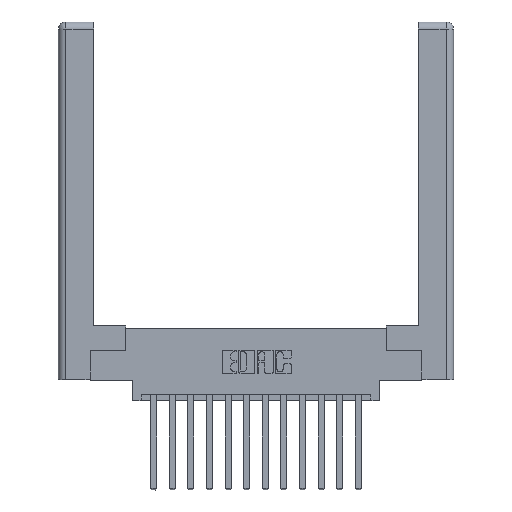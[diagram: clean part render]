
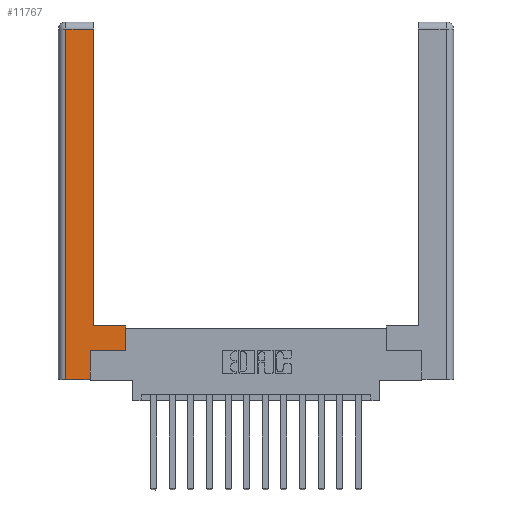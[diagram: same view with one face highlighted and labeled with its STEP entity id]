
A CAD part, top view. The second image highlights one B-rep face of the part: STEP entity #11767.
In plain terms, the highlighted planar face has unit normal (0, 0, 1).
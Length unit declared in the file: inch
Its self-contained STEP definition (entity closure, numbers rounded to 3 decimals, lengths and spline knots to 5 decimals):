
#79 = CARTESIAN_POINT ( 'NONE',  ( 0.265, 0.245, 0. ) ) ;
#194 = CARTESIAN_POINT ( 'NONE',  ( 0.295, 0.45, 0. ) ) ;
#247 = LINE ( 'NONE', #12439, #4839 ) ;
#283 = DIRECTION ( 'NONE',  ( -1., 0., 0. ) ) ;
#370 = LINE ( 'NONE', #435, #12954 ) ;
#431 = ORIENTED_EDGE ( 'NONE', *, *, #11980, .T. ) ;
#435 = CARTESIAN_POINT ( 'NONE',  ( 0.295, 3., 0. ) ) ;
#1293 = CARTESIAN_POINT ( 'NONE',  ( 0.565, 0.45, 0. ) ) ;
#1316 = CARTESIAN_POINT ( 'NONE',  ( 0.565, 0.245, 0. ) ) ;
#1406 = PLANE ( 'NONE',  #14299 ) ;
#1711 = VERTEX_POINT ( 'NONE', #15474 ) ;
#1734 = VERTEX_POINT ( 'NONE', #9394 ) ;
#1900 = CARTESIAN_POINT ( 'NONE',  ( 0.0615, 0., 0. ) ) ;
#2118 = CARTESIAN_POINT ( 'NONE',  ( 0.0615, 2.94, 0. ) ) ;
#2550 = DIRECTION ( 'NONE',  ( 1., 0., 0. ) ) ;
#3252 = CARTESIAN_POINT ( 'NONE',  ( 0.295, 2.94, 0. ) ) ;
#3367 = EDGE_CURVE ( 'NONE', #1734, #9697, #247, .T. ) ;
#4539 = VECTOR ( 'NONE', #8181, 39.37008 ) ;
#4839 = VECTOR ( 'NONE', #6400, 39.37008 ) ;
#5872 = VERTEX_POINT ( 'NONE', #3252 ) ;
#5894 = VECTOR ( 'NONE', #8075, 39.37008 ) ;
#6218 = EDGE_CURVE ( 'NONE', #12715, #5872, #370, .T. ) ;
#6400 = DIRECTION ( 'NONE',  ( 0., 1., 0. ) ) ;
#6417 = EDGE_CURVE ( 'NONE', #15620, #12715, #11399, .T. ) ;
#6690 = VERTEX_POINT ( 'NONE', #12395 ) ;
#6748 = EDGE_LOOP ( 'NONE', ( #7968, #11592, #431, #14269, #9908, #12900, #11451, #14509 ) ) ;
#6798 = FACE_OUTER_BOUND ( 'NONE', #6748, .T. ) ;
#6799 = EDGE_CURVE ( 'NONE', #9697, #1711, #15414, .T. ) ;
#7770 = LINE ( 'NONE', #2118, #4539 ) ;
#7968 = ORIENTED_EDGE ( 'NONE', *, *, #6218, .T. ) ;
#8075 = DIRECTION ( 'NONE',  ( 1., 0., 0. ) ) ;
#8181 = DIRECTION ( 'NONE',  ( -1., 0., 0. ) ) ;
#8554 = VECTOR ( 'NONE', #14557, 39.37008 ) ;
#8753 = DIRECTION ( 'NONE',  ( 0., 0., -1. ) ) ;
#9248 = LINE ( 'NONE', #1900, #11535 ) ;
#9306 = EDGE_CURVE ( 'NONE', #1711, #15620, #10464, .T. ) ;
#9394 = CARTESIAN_POINT ( 'NONE',  ( 0.265, 0., 0. ) ) ;
#9418 = EDGE_CURVE ( 'NONE', #14485, #1734, #11393, .T. ) ;
#9697 = VERTEX_POINT ( 'NONE', #79 ) ;
#9908 = ORIENTED_EDGE ( 'NONE', *, *, #3367, .T. ) ;
#10261 = VECTOR ( 'NONE', #14884, 39.37008 ) ;
#10464 = LINE ( 'NONE', #1293, #8554 ) ;
#10730 = CARTESIAN_POINT ( 'NONE',  ( 0.295, 0.45, 0. ) ) ;
#11196 = EDGE_CURVE ( 'NONE', #5872, #6690, #7770, .T. ) ;
#11241 = DIRECTION ( 'NONE',  ( 0., 1., 0. ) ) ;
#11393 = LINE ( 'NONE', #12591, #5894 ) ;
#11399 = LINE ( 'NONE', #194, #10261 ) ;
#11451 = ORIENTED_EDGE ( 'NONE', *, *, #9306, .T. ) ;
#11535 = VECTOR ( 'NONE', #11788, 39.37008 ) ;
#11592 = ORIENTED_EDGE ( 'NONE', *, *, #11196, .T. ) ;
#11767 = ADVANCED_FACE ( 'NONE', ( #6798 ), #1406, .F. ) ;
#11788 = DIRECTION ( 'NONE',  ( 0., -1., 0. ) ) ;
#11980 = EDGE_CURVE ( 'NONE', #6690, #14485, #9248, .T. ) ;
#12395 = CARTESIAN_POINT ( 'NONE',  ( 0.0615, 2.94, 0. ) ) ;
#12439 = CARTESIAN_POINT ( 'NONE',  ( 0.265, 0.245, 0. ) ) ;
#12563 = CARTESIAN_POINT ( 'NONE',  ( 0.565, 0.45, 0. ) ) ;
#12591 = CARTESIAN_POINT ( 'NONE',  ( 0.265, 0., 0. ) ) ;
#12715 = VERTEX_POINT ( 'NONE', #10730 ) ;
#12787 = CARTESIAN_POINT ( 'NONE',  ( 0.0615, 0., 0. ) ) ;
#12900 = ORIENTED_EDGE ( 'NONE', *, *, #6799, .T. ) ;
#12954 = VECTOR ( 'NONE', #11241, 39.37008 ) ;
#14269 = ORIENTED_EDGE ( 'NONE', *, *, #9418, .T. ) ;
#14299 = AXIS2_PLACEMENT_3D ( 'NONE', #14926, #8753, #283 ) ;
#14430 = VECTOR ( 'NONE', #2550, 39.37008 ) ;
#14485 = VERTEX_POINT ( 'NONE', #12787 ) ;
#14509 = ORIENTED_EDGE ( 'NONE', *, *, #6417, .T. ) ;
#14557 = DIRECTION ( 'NONE',  ( 0., 1., 0. ) ) ;
#14884 = DIRECTION ( 'NONE',  ( -1., 0., 0. ) ) ;
#14926 = CARTESIAN_POINT ( 'NONE',  ( 0., 0., 0. ) ) ;
#15414 = LINE ( 'NONE', #1316, #14430 ) ;
#15474 = CARTESIAN_POINT ( 'NONE',  ( 0.565, 0.245, 0. ) ) ;
#15620 = VERTEX_POINT ( 'NONE', #12563 ) ;
